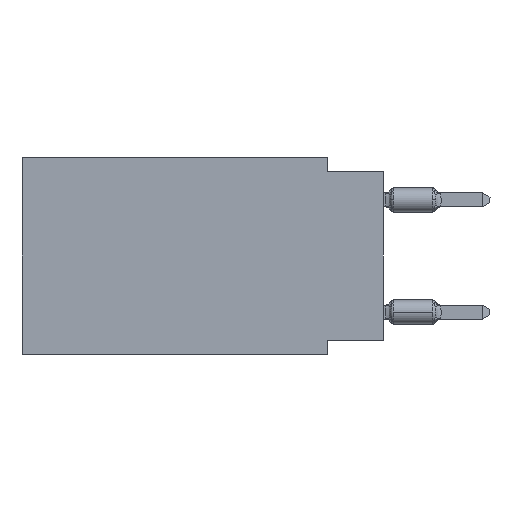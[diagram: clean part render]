
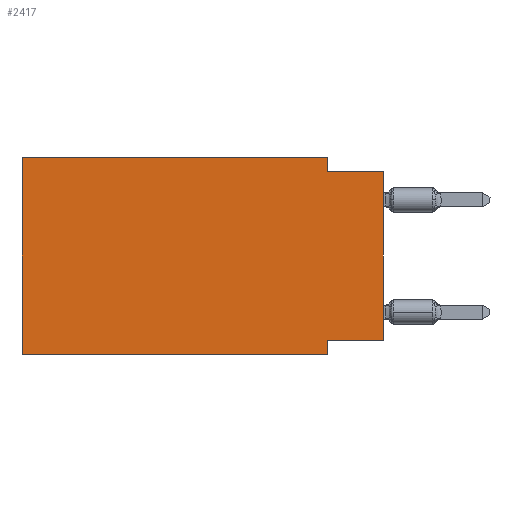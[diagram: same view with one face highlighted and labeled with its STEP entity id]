
A CAD part, left-side view. The second image highlights one B-rep face of the part: STEP entity #2417.
In plain terms, the highlighted planar face has unit normal (-1, 0, 0).
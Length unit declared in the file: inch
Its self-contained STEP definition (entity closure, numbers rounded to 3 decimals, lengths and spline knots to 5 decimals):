
#304 = CARTESIAN_POINT ( 'NONE',  ( 0., 0., -0.325 ) ) ;
#495 = ORIENTED_EDGE ( 'NONE', *, *, #10131, .F. ) ;
#898 = VECTOR ( 'NONE', #7649, 39.37008 ) ;
#1002 = VECTOR ( 'NONE', #1674, 39.37008 ) ;
#1080 = DIRECTION ( 'NONE',  ( 0., -1., 0. ) ) ;
#1659 = ORIENTED_EDGE ( 'NONE', *, *, #3262, .F. ) ;
#1674 = DIRECTION ( 'NONE',  ( 0., -1., 0. ) ) ;
#1763 = EDGE_CURVE ( 'NONE', #14953, #2191, #11327, .T. ) ;
#2191 = VERTEX_POINT ( 'NONE', #13372 ) ;
#2417 = ADVANCED_FACE ( 'NONE', ( #9382 ), #5696, .F. ) ;
#2866 = CARTESIAN_POINT ( 'NONE',  ( 0., 0.1, 0. ) ) ;
#3068 = EDGE_LOOP ( 'NONE', ( #12236, #6352, #5577, #1659, #11305, #9223, #495, #10088 ) ) ;
#3087 = LINE ( 'NONE', #12526, #1002 ) ;
#3238 = CARTESIAN_POINT ( 'NONE',  ( 0., 0.1, -0.35 ) ) ;
#3262 = EDGE_CURVE ( 'NONE', #9143, #14953, #4616, .T. ) ;
#3451 = VERTEX_POINT ( 'NONE', #5233 ) ;
#3638 = EDGE_CURVE ( 'NONE', #8363, #9143, #9226, .T. ) ;
#3940 = DIRECTION ( 'NONE',  ( 0., 1., 0. ) ) ;
#4201 = CARTESIAN_POINT ( 'NONE',  ( 0., 0.645, -0.35 ) ) ;
#4616 = LINE ( 'NONE', #9470, #13396 ) ;
#4680 = CARTESIAN_POINT ( 'NONE',  ( 0., 0.645, 0. ) ) ;
#4755 = VECTOR ( 'NONE', #6850, 39.37008 ) ;
#5233 = CARTESIAN_POINT ( 'NONE',  ( 0., 0., -0.325 ) ) ;
#5577 = ORIENTED_EDGE ( 'NONE', *, *, #1763, .F. ) ;
#5696 = PLANE ( 'NONE',  #10357 ) ;
#6278 = CARTESIAN_POINT ( 'NONE',  ( 0., 0.645, 0. ) ) ;
#6352 = ORIENTED_EDGE ( 'NONE', *, *, #15339, .F. ) ;
#6377 = LINE ( 'NONE', #304, #12941 ) ;
#6850 = DIRECTION ( 'NONE',  ( 0., 0., 1. ) ) ;
#7180 = LINE ( 'NONE', #8277, #7924 ) ;
#7379 = VECTOR ( 'NONE', #12704, 39.37008 ) ;
#7649 = DIRECTION ( 'NONE',  ( 0., 0., -1. ) ) ;
#7807 = CARTESIAN_POINT ( 'NONE',  ( 0., 0., 0. ) ) ;
#7924 = VECTOR ( 'NONE', #9583, 39.37008 ) ;
#8074 = DIRECTION ( 'NONE',  ( 0., 0., 1. ) ) ;
#8081 = VERTEX_POINT ( 'NONE', #3238 ) ;
#8277 = CARTESIAN_POINT ( 'NONE',  ( 0., 0.1, -0.35 ) ) ;
#8363 = VERTEX_POINT ( 'NONE', #12008 ) ;
#8454 = EDGE_CURVE ( 'NONE', #8363, #8081, #13800, .T. ) ;
#8894 = LINE ( 'NONE', #7807, #4755 ) ;
#9143 = VERTEX_POINT ( 'NONE', #6278 ) ;
#9223 = ORIENTED_EDGE ( 'NONE', *, *, #8454, .T. ) ;
#9226 = LINE ( 'NONE', #11677, #13692 ) ;
#9382 = FACE_OUTER_BOUND ( 'NONE', #3068, .T. ) ;
#9470 = CARTESIAN_POINT ( 'NONE',  ( 0., 0.645, 0. ) ) ;
#9583 = DIRECTION ( 'NONE',  ( 0., 0., -1. ) ) ;
#10088 = ORIENTED_EDGE ( 'NONE', *, *, #10264, .F. ) ;
#10131 = EDGE_CURVE ( 'NONE', #13437, #8081, #7180, .T. ) ;
#10264 = EDGE_CURVE ( 'NONE', #3451, #13437, #6377, .T. ) ;
#10357 = AXIS2_PLACEMENT_3D ( 'NONE', #4680, #15291, #11592 ) ;
#10394 = CARTESIAN_POINT ( 'NONE',  ( 0., 0.1, 0. ) ) ;
#11305 = ORIENTED_EDGE ( 'NONE', *, *, #3638, .F. ) ;
#11327 = LINE ( 'NONE', #2866, #898 ) ;
#11568 = VERTEX_POINT ( 'NONE', #11710 ) ;
#11592 = DIRECTION ( 'NONE',  ( 0., 0., -1. ) ) ;
#11677 = CARTESIAN_POINT ( 'NONE',  ( 0., 0.645, 0. ) ) ;
#11710 = CARTESIAN_POINT ( 'NONE',  ( 0., 0., -0.025 ) ) ;
#12008 = CARTESIAN_POINT ( 'NONE',  ( 0., 0.645, -0.35 ) ) ;
#12236 = ORIENTED_EDGE ( 'NONE', *, *, #12776, .T. ) ;
#12526 = CARTESIAN_POINT ( 'NONE',  ( 0., 0., -0.025 ) ) ;
#12704 = DIRECTION ( 'NONE',  ( 0., -1., 0. ) ) ;
#12776 = EDGE_CURVE ( 'NONE', #3451, #11568, #8894, .T. ) ;
#12941 = VECTOR ( 'NONE', #3940, 39.37008 ) ;
#13372 = CARTESIAN_POINT ( 'NONE',  ( 0., 0.1, -0.025 ) ) ;
#13396 = VECTOR ( 'NONE', #1080, 39.37008 ) ;
#13437 = VERTEX_POINT ( 'NONE', #15468 ) ;
#13692 = VECTOR ( 'NONE', #8074, 39.37008 ) ;
#13800 = LINE ( 'NONE', #4201, #7379 ) ;
#14953 = VERTEX_POINT ( 'NONE', #10394 ) ;
#15291 = DIRECTION ( 'NONE',  ( 1., 0., 0. ) ) ;
#15339 = EDGE_CURVE ( 'NONE', #2191, #11568, #3087, .T. ) ;
#15468 = CARTESIAN_POINT ( 'NONE',  ( 0., 0.1, -0.325 ) ) ;
